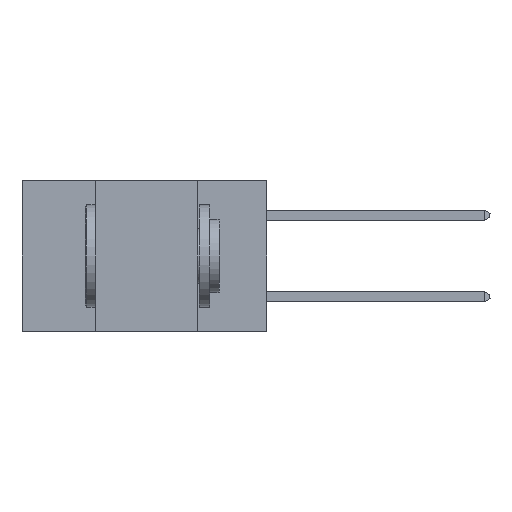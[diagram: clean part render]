
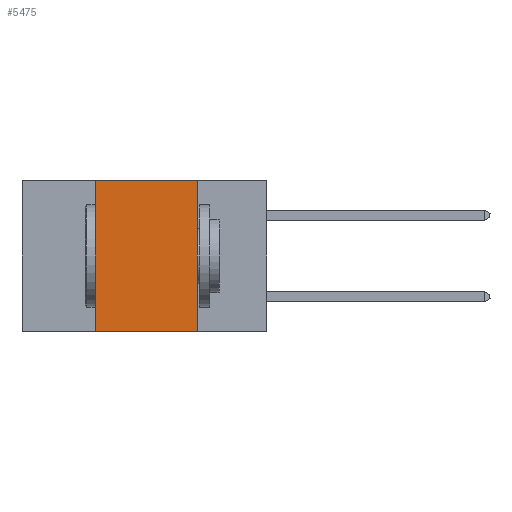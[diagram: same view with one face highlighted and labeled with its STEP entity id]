
A CAD part, left-side view. The second image highlights one B-rep face of the part: STEP entity #5475.
In plain terms, the highlighted planar face has unit normal (-1, 0, 0).
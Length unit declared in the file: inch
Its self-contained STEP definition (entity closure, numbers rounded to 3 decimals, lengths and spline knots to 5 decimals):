
#284 = EDGE_LOOP ( 'NONE', ( #15224, #10062, #30609, #25686 ) ) ;
#539 = LINE ( 'NONE', #2034, #26542 ) ;
#2034 = CARTESIAN_POINT ( 'NONE',  ( 0., 0.42, 0. ) ) ;
#2659 = CARTESIAN_POINT ( 'NONE',  ( 0., 0.17, -0.37 ) ) ;
#3256 = LINE ( 'NONE', #14698, #29089 ) ;
#4323 = CARTESIAN_POINT ( 'NONE',  ( 0., 0.42, 0. ) ) ;
#4722 = LINE ( 'NONE', #9744, #17479 ) ;
#5475 = ADVANCED_FACE ( 'NONE', ( #12391 ), #26941, .F. ) ;
#7283 = LINE ( 'NONE', #26813, #32222 ) ;
#9703 = DIRECTION ( 'NONE',  ( 0., 0., -1. ) ) ;
#9744 = CARTESIAN_POINT ( 'NONE',  ( 0., 0.6, -0.37 ) ) ;
#10062 = ORIENTED_EDGE ( 'NONE', *, *, #13155, .F. ) ;
#12391 = FACE_OUTER_BOUND ( 'NONE', #284, .T. ) ;
#13155 = EDGE_CURVE ( 'NONE', #19895, #19564, #7283, .T. ) ;
#13264 = CARTESIAN_POINT ( 'NONE',  ( 0., 0.17, 0. ) ) ;
#13426 = VERTEX_POINT ( 'NONE', #2659 ) ;
#14639 = DIRECTION ( 'NONE',  ( 1., 0., 0. ) ) ;
#14698 = CARTESIAN_POINT ( 'NONE',  ( 0., 0.17, 0. ) ) ;
#15224 = ORIENTED_EDGE ( 'NONE', *, *, #19970, .F. ) ;
#15572 = VERTEX_POINT ( 'NONE', #22564 ) ;
#17479 = VECTOR ( 'NONE', #27146, 39.37008 ) ;
#19564 = VERTEX_POINT ( 'NONE', #13264 ) ;
#19895 = VERTEX_POINT ( 'NONE', #4323 ) ;
#19970 = EDGE_CURVE ( 'NONE', #19564, #13426, #3256, .T. ) ;
#20555 = AXIS2_PLACEMENT_3D ( 'NONE', #29374, #14639, #31873 ) ;
#22564 = CARTESIAN_POINT ( 'NONE',  ( 0., 0.42, -0.37 ) ) ;
#22742 = EDGE_CURVE ( 'NONE', #15572, #13426, #4722, .T. ) ;
#25686 = ORIENTED_EDGE ( 'NONE', *, *, #22742, .T. ) ;
#26542 = VECTOR ( 'NONE', #27181, 39.37008 ) ;
#26813 = CARTESIAN_POINT ( 'NONE',  ( 0., 0.6, 0. ) ) ;
#26941 = PLANE ( 'NONE',  #20555 ) ;
#27039 = EDGE_CURVE ( 'NONE', #15572, #19895, #539, .T. ) ;
#27146 = DIRECTION ( 'NONE',  ( 0., -1., 0. ) ) ;
#27181 = DIRECTION ( 'NONE',  ( 0., 0., 1. ) ) ;
#29089 = VECTOR ( 'NONE', #9703, 39.37008 ) ;
#29243 = DIRECTION ( 'NONE',  ( 0., -1., 0. ) ) ;
#29374 = CARTESIAN_POINT ( 'NONE',  ( 0., 0.6, 0. ) ) ;
#30609 = ORIENTED_EDGE ( 'NONE', *, *, #27039, .F. ) ;
#31873 = DIRECTION ( 'NONE',  ( 0., 0., -1. ) ) ;
#32222 = VECTOR ( 'NONE', #29243, 39.37008 ) ;
